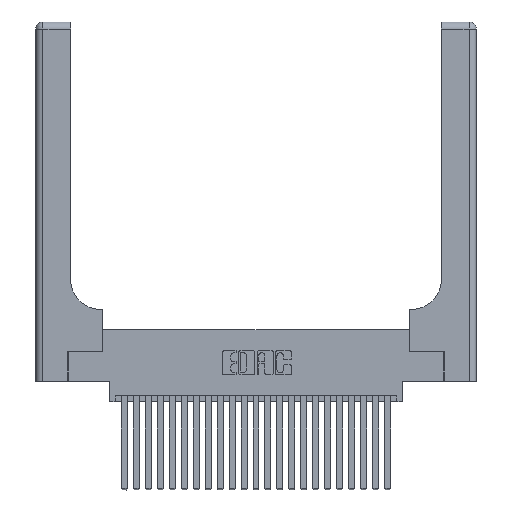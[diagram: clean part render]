
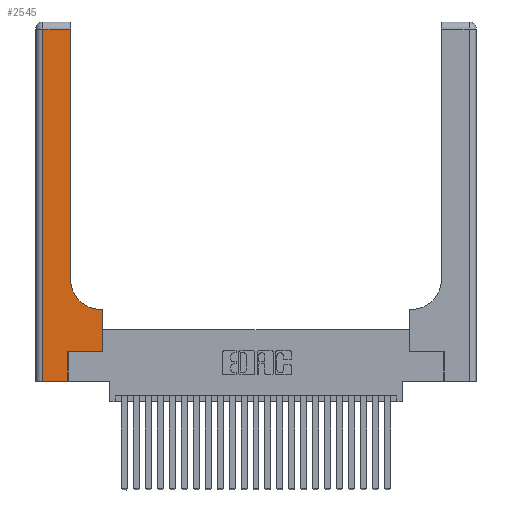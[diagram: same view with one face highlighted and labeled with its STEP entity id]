
A CAD part, top view. The second image highlights one B-rep face of the part: STEP entity #2545.
In plain terms, the highlighted planar face has unit normal (0, 0, 1).
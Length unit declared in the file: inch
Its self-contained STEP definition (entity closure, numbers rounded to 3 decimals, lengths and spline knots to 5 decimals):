
#299 = CARTESIAN_POINT ( 'NONE',  ( 0.2915, 0.6, 0.37 ) ) ;
#400 = DIRECTION ( 'NONE',  ( 0., 1., 0. ) ) ;
#420 = CARTESIAN_POINT ( 'NONE',  ( 0.269, 0., 0.37 ) ) ;
#501 = VECTOR ( 'NONE', #12939, 39.37008 ) ;
#760 = VECTOR ( 'NONE', #8141, 39.37008 ) ;
#791 = CARTESIAN_POINT ( 'NONE',  ( 0.269, 0.25, 0.37 ) ) ;
#1376 = VECTOR ( 'NONE', #18589, 39.37008 ) ;
#2073 = ORIENTED_EDGE ( 'NONE', *, *, #3219, .T. ) ;
#2545 = ADVANCED_FACE ( 'NONE', ( #19119 ), #22674, .F. ) ;
#2571 = DIRECTION ( 'NONE',  ( 1., 0., 0. ) ) ;
#2836 = DIRECTION ( 'NONE',  ( 0., 0., -1. ) ) ;
#2864 = ORIENTED_EDGE ( 'NONE', *, *, #5341, .T. ) ;
#2996 = CARTESIAN_POINT ( 'NONE',  ( 0., 2.94, 0.37 ) ) ;
#3219 = EDGE_CURVE ( 'NONE', #19381, #13154, #20941, .T. ) ;
#3510 = ORIENTED_EDGE ( 'NONE', *, *, #10625, .T. ) ;
#3708 = VECTOR ( 'NONE', #25543, 39.37008 ) ;
#4612 = AXIS2_PLACEMENT_3D ( 'NONE', #10786, #20686, #12037 ) ;
#4938 = EDGE_CURVE ( 'NONE', #16592, #5243, #15329, .T. ) ;
#5243 = VERTEX_POINT ( 'NONE', #20109 ) ;
#5341 = EDGE_CURVE ( 'NONE', #5243, #19381, #13744, .T. ) ;
#5930 = VERTEX_POINT ( 'NONE', #6044 ) ;
#6044 = CARTESIAN_POINT ( 'NONE',  ( 0.2915, 0.85, 0.37 ) ) ;
#6776 = LINE ( 'NONE', #23100, #10495 ) ;
#7110 = CARTESIAN_POINT ( 'NONE',  ( 0.5415, 0.6, 0.37 ) ) ;
#7524 = VECTOR ( 'NONE', #8198, 39.37008 ) ;
#7834 = ORIENTED_EDGE ( 'NONE', *, *, #15892, .T. ) ;
#8141 = DIRECTION ( 'NONE',  ( 0., 1., 0. ) ) ;
#8198 = DIRECTION ( 'NONE',  ( 0., -1., 0. ) ) ;
#8425 = CARTESIAN_POINT ( 'NONE',  ( 0., 0., 0.37 ) ) ;
#8536 = CARTESIAN_POINT ( 'NONE',  ( 0.269, 0., 0.37 ) ) ;
#8589 = VERTEX_POINT ( 'NONE', #23490 ) ;
#9900 = VERTEX_POINT ( 'NONE', #18438 ) ;
#9901 = ORIENTED_EDGE ( 'NONE', *, *, #15611, .T. ) ;
#10158 = VERTEX_POINT ( 'NONE', #14416 ) ;
#10351 = VECTOR ( 'NONE', #21979, 39.37008 ) ;
#10378 = ORIENTED_EDGE ( 'NONE', *, *, #16541, .T. ) ;
#10436 = LINE ( 'NONE', #2996, #501 ) ;
#10495 = VECTOR ( 'NONE', #400, 39.37008 ) ;
#10625 = EDGE_CURVE ( 'NONE', #10158, #16592, #10436, .T. ) ;
#10786 = CARTESIAN_POINT ( 'NONE',  ( 0., 3., 0.37 ) ) ;
#11390 = VECTOR ( 'NONE', #19639, 39.37008 ) ;
#12037 = DIRECTION ( 'NONE',  ( -1., 0., 0. ) ) ;
#12939 = DIRECTION ( 'NONE',  ( -1., 0., 0. ) ) ;
#13154 = VERTEX_POINT ( 'NONE', #791 ) ;
#13744 = LINE ( 'NONE', #8425, #1376 ) ;
#14200 = VERTEX_POINT ( 'NONE', #7110 ) ;
#14416 = CARTESIAN_POINT ( 'NONE',  ( 0.2915, 2.94, 0.37 ) ) ;
#14945 = EDGE_CURVE ( 'NONE', #13154, #9900, #20803, .T. ) ;
#15329 = LINE ( 'NONE', #19339, #7524 ) ;
#15611 = EDGE_CURVE ( 'NONE', #9900, #8589, #6776, .T. ) ;
#15892 = EDGE_CURVE ( 'NONE', #14200, #5930, #21052, .T. ) ;
#15952 = LINE ( 'NONE', #299, #10351 ) ;
#16541 = EDGE_CURVE ( 'NONE', #5930, #10158, #19469, .T. ) ;
#16592 = VERTEX_POINT ( 'NONE', #19309 ) ;
#17540 = CARTESIAN_POINT ( 'NONE',  ( 0.269, 0.25, 0.37 ) ) ;
#18438 = CARTESIAN_POINT ( 'NONE',  ( 0.5585, 0.25, 0.37 ) ) ;
#18589 = DIRECTION ( 'NONE',  ( 1., 0., 0. ) ) ;
#19119 = FACE_OUTER_BOUND ( 'NONE', #19772, .T. ) ;
#19309 = CARTESIAN_POINT ( 'NONE',  ( 0.06, 2.94, 0.37 ) ) ;
#19339 = CARTESIAN_POINT ( 'NONE',  ( 0.06, 3., 0.37 ) ) ;
#19381 = VERTEX_POINT ( 'NONE', #8536 ) ;
#19469 = LINE ( 'NONE', #23394, #11390 ) ;
#19639 = DIRECTION ( 'NONE',  ( 0., 1., 0. ) ) ;
#19772 = EDGE_LOOP ( 'NONE', ( #10378, #3510, #20210, #2864, #2073, #19923, #9901, #21521, #7834 ) ) ;
#19923 = ORIENTED_EDGE ( 'NONE', *, *, #14945, .T. ) ;
#20109 = CARTESIAN_POINT ( 'NONE',  ( 0.06, 0., 0.37 ) ) ;
#20198 = AXIS2_PLACEMENT_3D ( 'NONE', #22797, #2836, #2571 ) ;
#20210 = ORIENTED_EDGE ( 'NONE', *, *, #4938, .T. ) ;
#20686 = DIRECTION ( 'NONE',  ( 0., 0., -1. ) ) ;
#20803 = LINE ( 'NONE', #17540, #3708 ) ;
#20941 = LINE ( 'NONE', #420, #760 ) ;
#21052 = CIRCLE ( 'NONE', #20198, 0.25 ) ;
#21521 = ORIENTED_EDGE ( 'NONE', *, *, #22151, .T. ) ;
#21979 = DIRECTION ( 'NONE',  ( -1., 0., 0. ) ) ;
#22151 = EDGE_CURVE ( 'NONE', #8589, #14200, #15952, .T. ) ;
#22674 = PLANE ( 'NONE',  #4612 ) ;
#22797 = CARTESIAN_POINT ( 'NONE',  ( 0.5415, 0.85, 0.37 ) ) ;
#23100 = CARTESIAN_POINT ( 'NONE',  ( 0.5585, 0.25, 0.37 ) ) ;
#23394 = CARTESIAN_POINT ( 'NONE',  ( 0.2915, 3., 0.37 ) ) ;
#23490 = CARTESIAN_POINT ( 'NONE',  ( 0.5585, 0.6, 0.37 ) ) ;
#25543 = DIRECTION ( 'NONE',  ( 1., 0., 0. ) ) ;
